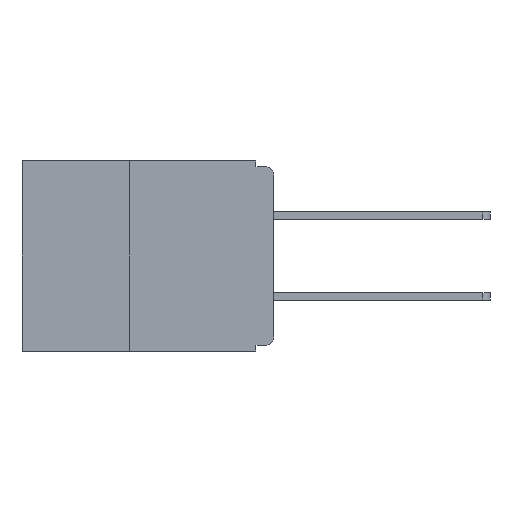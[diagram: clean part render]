
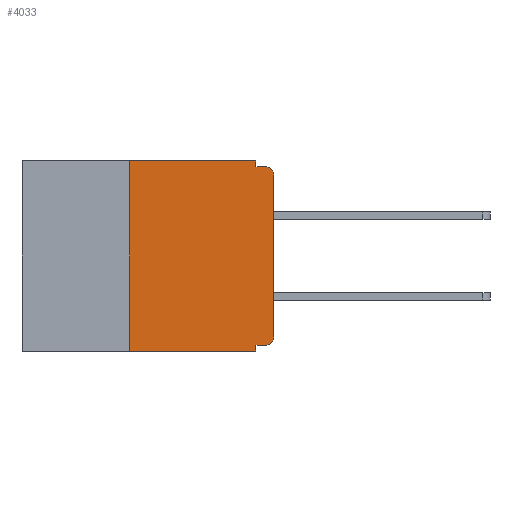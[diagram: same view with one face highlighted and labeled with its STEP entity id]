
A CAD part, left-side view. The second image highlights one B-rep face of the part: STEP entity #4033.
In plain terms, the highlighted planar face has unit normal (-1, 0, 0).
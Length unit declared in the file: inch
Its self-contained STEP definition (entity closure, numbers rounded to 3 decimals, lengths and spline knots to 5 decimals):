
#341 = ORIENTED_EDGE ( 'NONE', *, *, #9542, .T. ) ;
#614 = LINE ( 'NONE', #13937, #6762 ) ;
#897 = ORIENTED_EDGE ( 'NONE', *, *, #12279, .F. ) ;
#905 = CARTESIAN_POINT ( 'NONE',  ( 0., 0.25, -0.33 ) ) ;
#1277 = VECTOR ( 'NONE', #7988, 39.37008 ) ;
#1379 = CARTESIAN_POINT ( 'NONE',  ( 0., 0., -0.305 ) ) ;
#1635 = ORIENTED_EDGE ( 'NONE', *, *, #11719, .F. ) ;
#1636 = LINE ( 'NONE', #2672, #1277 ) ;
#1645 = AXIS2_PLACEMENT_3D ( 'NONE', #5925, #13760, #7090 ) ;
#1667 = CARTESIAN_POINT ( 'NONE',  ( 0., 0.015, -0.01 ) ) ;
#1823 = LINE ( 'NONE', #9078, #7615 ) ;
#2141 = CARTESIAN_POINT ( 'NONE',  ( 0., 0.015, -0.32 ) ) ;
#2161 = VECTOR ( 'NONE', #12311, 39.37008 ) ;
#2339 = EDGE_CURVE ( 'NONE', #14210, #7147, #5322, .T. ) ;
#2672 = CARTESIAN_POINT ( 'NONE',  ( 0., 0., 0. ) ) ;
#2703 = CARTESIAN_POINT ( 'NONE',  ( 0., 0.25, -0.33 ) ) ;
#2845 = VERTEX_POINT ( 'NONE', #10396 ) ;
#3115 = EDGE_CURVE ( 'NONE', #13718, #8562, #614, .T. ) ;
#3635 = EDGE_CURVE ( 'NONE', #13718, #14347, #12013, .T. ) ;
#4033 = ADVANCED_FACE ( 'NONE', ( #9717 ), #12660, .F. ) ;
#4195 = CARTESIAN_POINT ( 'NONE',  ( 0., 0.015, -0.025 ) ) ;
#4387 = CARTESIAN_POINT ( 'NONE',  ( 0., 0.031, 0. ) ) ;
#4481 = CARTESIAN_POINT ( 'NONE',  ( 0., 0.437, 0. ) ) ;
#4650 = CIRCLE ( 'NONE', #8290, 0.015 ) ;
#5017 = ORIENTED_EDGE ( 'NONE', *, *, #11745, .F. ) ;
#5155 = EDGE_CURVE ( 'NONE', #5424, #5883, #1636, .T. ) ;
#5322 = LINE ( 'NONE', #8890, #8729 ) ;
#5352 = EDGE_CURVE ( 'NONE', #11666, #2845, #13170, .T. ) ;
#5353 = DIRECTION ( 'NONE',  ( 0., 0., -1. ) ) ;
#5424 = VERTEX_POINT ( 'NONE', #1379 ) ;
#5883 = VERTEX_POINT ( 'NONE', #12152 ) ;
#5925 = CARTESIAN_POINT ( 'NONE',  ( 0., 0.015, -0.305 ) ) ;
#6548 = VECTOR ( 'NONE', #8039, 39.37008 ) ;
#6762 = VECTOR ( 'NONE', #8705, 39.37008 ) ;
#6835 = EDGE_LOOP ( 'NONE', ( #12623, #12803, #897, #9317, #1635, #12334, #8833, #5017, #10358, #341 ) ) ;
#6887 = LINE ( 'NONE', #6894, #6548 ) ;
#6894 = CARTESIAN_POINT ( 'NONE',  ( 0., 0., -0.01 ) ) ;
#7090 = DIRECTION ( 'NONE',  ( 0., 0., -1. ) ) ;
#7112 = AXIS2_PLACEMENT_3D ( 'NONE', #14072, #13274, #13227 ) ;
#7147 = VERTEX_POINT ( 'NONE', #9530 ) ;
#7615 = VECTOR ( 'NONE', #7959, 39.37008 ) ;
#7959 = DIRECTION ( 'NONE',  ( 0., 0., -1. ) ) ;
#7988 = DIRECTION ( 'NONE',  ( 0., 0., 1. ) ) ;
#8039 = DIRECTION ( 'NONE',  ( 0., -1., 0. ) ) ;
#8164 = VERTEX_POINT ( 'NONE', #1667 ) ;
#8290 = AXIS2_PLACEMENT_3D ( 'NONE', #4195, #12130, #5353 ) ;
#8562 = VERTEX_POINT ( 'NONE', #8619 ) ;
#8619 = CARTESIAN_POINT ( 'NONE',  ( 0., 0.031, -0.33 ) ) ;
#8705 = DIRECTION ( 'NONE',  ( 0., -1., 0. ) ) ;
#8729 = VECTOR ( 'NONE', #9271, 39.37008 ) ;
#8833 = ORIENTED_EDGE ( 'NONE', *, *, #3115, .T. ) ;
#8890 = CARTESIAN_POINT ( 'NONE',  ( 0., 0., -0.32 ) ) ;
#8905 = CIRCLE ( 'NONE', #1645, 0.015 ) ;
#9078 = CARTESIAN_POINT ( 'NONE',  ( 0., 0.031, -0.33 ) ) ;
#9271 = DIRECTION ( 'NONE',  ( 0., 1., 0. ) ) ;
#9317 = ORIENTED_EDGE ( 'NONE', *, *, #5352, .F. ) ;
#9530 = CARTESIAN_POINT ( 'NONE',  ( 0., 0.031, -0.32 ) ) ;
#9542 = EDGE_CURVE ( 'NONE', #14210, #5424, #8905, .T. ) ;
#9717 = FACE_OUTER_BOUND ( 'NONE', #6835, .T. ) ;
#10240 = VECTOR ( 'NONE', #12384, 39.37008 ) ;
#10358 = ORIENTED_EDGE ( 'NONE', *, *, #2339, .F. ) ;
#10396 = CARTESIAN_POINT ( 'NONE',  ( 0., 0.031, -0.01 ) ) ;
#11006 = DIRECTION ( 'NONE',  ( 0., 0., 1. ) ) ;
#11307 = LINE ( 'NONE', #4481, #2161 ) ;
#11666 = VERTEX_POINT ( 'NONE', #4387 ) ;
#11719 = EDGE_CURVE ( 'NONE', #14347, #11666, #11307, .T. ) ;
#11745 = EDGE_CURVE ( 'NONE', #7147, #8562, #1823, .T. ) ;
#12013 = LINE ( 'NONE', #905, #14533 ) ;
#12130 = DIRECTION ( 'NONE',  ( -1., 0., 0. ) ) ;
#12152 = CARTESIAN_POINT ( 'NONE',  ( 0., 0., -0.025 ) ) ;
#12279 = EDGE_CURVE ( 'NONE', #2845, #8164, #6887, .T. ) ;
#12311 = DIRECTION ( 'NONE',  ( 0., -1., 0. ) ) ;
#12334 = ORIENTED_EDGE ( 'NONE', *, *, #3635, .F. ) ;
#12384 = DIRECTION ( 'NONE',  ( 0., 0., -1. ) ) ;
#12623 = ORIENTED_EDGE ( 'NONE', *, *, #5155, .T. ) ;
#12653 = CARTESIAN_POINT ( 'NONE',  ( 0., 0.25, 0. ) ) ;
#12660 = PLANE ( 'NONE',  #7112 ) ;
#12803 = ORIENTED_EDGE ( 'NONE', *, *, #13276, .T. ) ;
#12893 = CARTESIAN_POINT ( 'NONE',  ( 0., 0.031, 0. ) ) ;
#13170 = LINE ( 'NONE', #12893, #10240 ) ;
#13227 = DIRECTION ( 'NONE',  ( 0., 0., -1. ) ) ;
#13274 = DIRECTION ( 'NONE',  ( 1., 0., 0. ) ) ;
#13276 = EDGE_CURVE ( 'NONE', #5883, #8164, #4650, .T. ) ;
#13718 = VERTEX_POINT ( 'NONE', #2703 ) ;
#13760 = DIRECTION ( 'NONE',  ( -1., 0., 0. ) ) ;
#13937 = CARTESIAN_POINT ( 'NONE',  ( 0., 0.437, -0.33 ) ) ;
#14072 = CARTESIAN_POINT ( 'NONE',  ( 0., 0.437, 0. ) ) ;
#14210 = VERTEX_POINT ( 'NONE', #2141 ) ;
#14347 = VERTEX_POINT ( 'NONE', #12653 ) ;
#14533 = VECTOR ( 'NONE', #11006, 39.37008 ) ;
